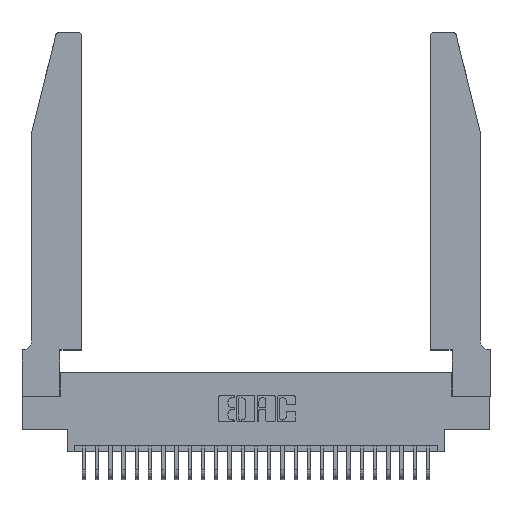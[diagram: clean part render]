
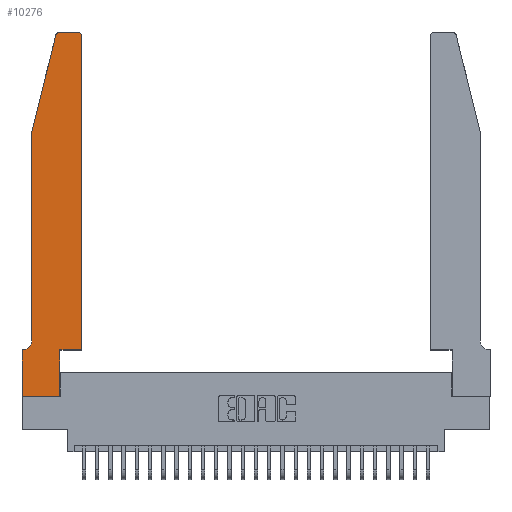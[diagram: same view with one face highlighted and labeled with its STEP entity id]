
A CAD part, top view. The second image highlights one B-rep face of the part: STEP entity #10276.
In plain terms, the highlighted planar face has unit normal (0, 0, 1).
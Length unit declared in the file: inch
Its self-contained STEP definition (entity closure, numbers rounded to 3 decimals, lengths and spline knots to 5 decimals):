
#177 = EDGE_CURVE ( 'NONE', #12363, #7937, #10976, .T. ) ;
#360 = DIRECTION ( 'NONE',  ( 0., -1., 0. ) ) ;
#471 = CARTESIAN_POINT ( 'NONE',  ( 0., 0., 0.37 ) ) ;
#489 = VERTEX_POINT ( 'NONE', #28888 ) ;
#688 = DIRECTION ( 'NONE',  ( -0.239, -0.971, 0. ) ) ;
#980 = EDGE_CURVE ( 'NONE', #6203, #19914, #10920, .T. ) ;
#1013 = CARTESIAN_POINT ( 'NONE',  ( 0., 0., 0.37 ) ) ;
#1745 = CARTESIAN_POINT ( 'NONE',  ( 0.4505, 0.35, 0.37 ) ) ;
#2110 = EDGE_CURVE ( 'NONE', #11754, #8793, #12987, .T. ) ;
#2292 = CARTESIAN_POINT ( 'NONE',  ( 0.0755, 2., 0.37 ) ) ;
#2391 = VERTEX_POINT ( 'NONE', #14574 ) ;
#2503 = VECTOR ( 'NONE', #2788, 39.37008 ) ;
#2513 = ORIENTED_EDGE ( 'NONE', *, *, #2110, .T. ) ;
#2583 = ORIENTED_EDGE ( 'NONE', *, *, #15632, .T. ) ;
#2654 = EDGE_CURVE ( 'NONE', #11881, #7497, #23380, .T. ) ;
#2788 = DIRECTION ( 'NONE',  ( -1., 0., 0. ) ) ;
#2867 = VECTOR ( 'NONE', #21443, 39.37008 ) ;
#3719 = DIRECTION ( 'NONE',  ( 0., 0., 1. ) ) ;
#3841 = CARTESIAN_POINT ( 'NONE',  ( 0.4205, 2.75, 0.37 ) ) ;
#4377 = VECTOR ( 'NONE', #18236, 39.37008 ) ;
#4648 = CARTESIAN_POINT ( 'NONE',  ( 0.284, 2.72, 0.37 ) ) ;
#5442 = DIRECTION ( 'NONE',  ( 1., 0., 0. ) ) ;
#5841 = CARTESIAN_POINT ( 'NONE',  ( 0., 0.35, 0.37 ) ) ;
#6203 = VERTEX_POINT ( 'NONE', #15673 ) ;
#6732 = VECTOR ( 'NONE', #360, 39.37008 ) ;
#6877 = VECTOR ( 'NONE', #18869, 39.37008 ) ;
#7497 = VERTEX_POINT ( 'NONE', #13960 ) ;
#7697 = CARTESIAN_POINT ( 'NONE',  ( 0.0755, 0.42, 0.37 ) ) ;
#7933 = CARTESIAN_POINT ( 'NONE',  ( 0.4205, 2.72, 0.37 ) ) ;
#7937 = VERTEX_POINT ( 'NONE', #13743 ) ;
#8663 = FACE_OUTER_BOUND ( 'NONE', #11438, .T. ) ;
#8793 = VERTEX_POINT ( 'NONE', #24469 ) ;
#9439 = LINE ( 'NONE', #27641, #4377 ) ;
#9674 = DIRECTION ( 'NONE',  ( 0., -1., 0. ) ) ;
#9927 = CARTESIAN_POINT ( 'NONE',  ( 0.4505, 0.35, 0.37 ) ) ;
#9964 = ORIENTED_EDGE ( 'NONE', *, *, #21412, .T. ) ;
#10276 = ADVANCED_FACE ( 'NONE', ( #8663 ), #26796, .T. ) ;
#10920 = LINE ( 'NONE', #14162, #12717 ) ;
#10976 = CIRCLE ( 'NONE', #28673, 0.07 ) ;
#11080 = VERTEX_POINT ( 'NONE', #28340 ) ;
#11148 = ORIENTED_EDGE ( 'NONE', *, *, #28924, .T. ) ;
#11221 = EDGE_CURVE ( 'NONE', #7937, #2391, #26223, .T. ) ;
#11438 = EDGE_LOOP ( 'NONE', ( #2513, #26352, #26016, #28438, #24859, #29668, #17310, #9964, #19159, #11148, #24002, #2583 ) ) ;
#11528 = LINE ( 'NONE', #12059, #2867 ) ;
#11667 = DIRECTION ( 'NONE',  ( 1., 0., 0. ) ) ;
#11708 = DIRECTION ( 'NONE',  ( 0., 0., -1. ) ) ;
#11754 = VERTEX_POINT ( 'NONE', #3841 ) ;
#11881 = VERTEX_POINT ( 'NONE', #9927 ) ;
#11936 = AXIS2_PLACEMENT_3D ( 'NONE', #7933, #19351, #29120 ) ;
#12022 = CARTESIAN_POINT ( 'NONE',  ( 0.2605, 2.75, 0.37 ) ) ;
#12059 = CARTESIAN_POINT ( 'NONE',  ( 0.4505, 0.35, 0.37 ) ) ;
#12363 = VERTEX_POINT ( 'NONE', #7697 ) ;
#12428 = CIRCLE ( 'NONE', #14003, 0.03 ) ;
#12717 = VECTOR ( 'NONE', #688, 39.37008 ) ;
#12831 = LINE ( 'NONE', #471, #6732 ) ;
#12987 = LINE ( 'NONE', #12022, #6877 ) ;
#13413 = EDGE_CURVE ( 'NONE', #8793, #6203, #12428, .T. ) ;
#13743 = CARTESIAN_POINT ( 'NONE',  ( 0.0055, 0.35, 0.37 ) ) ;
#13960 = CARTESIAN_POINT ( 'NONE',  ( 0.4505, 2.72, 0.37 ) ) ;
#14003 = AXIS2_PLACEMENT_3D ( 'NONE', #4648, #18229, #11667 ) ;
#14131 = DIRECTION ( 'NONE',  ( -1., 0., 0. ) ) ;
#14162 = CARTESIAN_POINT ( 'NONE',  ( 0.0755, 2., 0.37 ) ) ;
#14574 = CARTESIAN_POINT ( 'NONE',  ( 0., 0.35, 0.37 ) ) ;
#15402 = EDGE_CURVE ( 'NONE', #25795, #11080, #9439, .T. ) ;
#15632 = EDGE_CURVE ( 'NONE', #7497, #11754, #22418, .T. ) ;
#15673 = CARTESIAN_POINT ( 'NONE',  ( 0.25487, 2.72718, 0.37 ) ) ;
#16057 = CARTESIAN_POINT ( 'NONE',  ( 0.0055, 0.42, 0.37 ) ) ;
#16562 = CARTESIAN_POINT ( 'NONE',  ( 0.0755, 0.35, 0.37 ) ) ;
#16608 = LINE ( 'NONE', #1013, #21671 ) ;
#17310 = ORIENTED_EDGE ( 'NONE', *, *, #24957, .T. ) ;
#17913 = CARTESIAN_POINT ( 'NONE',  ( 0.2865, 0., 0.37 ) ) ;
#18229 = DIRECTION ( 'NONE',  ( 0., 0., 1. ) ) ;
#18236 = DIRECTION ( 'NONE',  ( 0., 1., 0. ) ) ;
#18338 = LINE ( 'NONE', #25824, #28359 ) ;
#18869 = DIRECTION ( 'NONE',  ( -1., 0., 0. ) ) ;
#19159 = ORIENTED_EDGE ( 'NONE', *, *, #15402, .T. ) ;
#19351 = DIRECTION ( 'NONE',  ( 0., 0., 1. ) ) ;
#19914 = VERTEX_POINT ( 'NONE', #2292 ) ;
#21412 = EDGE_CURVE ( 'NONE', #489, #25795, #16608, .T. ) ;
#21443 = DIRECTION ( 'NONE',  ( 1., 0., 0. ) ) ;
#21671 = VECTOR ( 'NONE', #5442, 39.37008 ) ;
#22418 = CIRCLE ( 'NONE', #11936, 0.03 ) ;
#22507 = EDGE_CURVE ( 'NONE', #19914, #12363, #18338, .T. ) ;
#23380 = LINE ( 'NONE', #1745, #27680 ) ;
#24002 = ORIENTED_EDGE ( 'NONE', *, *, #2654, .T. ) ;
#24469 = CARTESIAN_POINT ( 'NONE',  ( 0.284, 2.75, 0.37 ) ) ;
#24859 = ORIENTED_EDGE ( 'NONE', *, *, #177, .T. ) ;
#24957 = EDGE_CURVE ( 'NONE', #2391, #489, #12831, .T. ) ;
#25778 = AXIS2_PLACEMENT_3D ( 'NONE', #5841, #3719, #28824 ) ;
#25795 = VERTEX_POINT ( 'NONE', #17913 ) ;
#25824 = CARTESIAN_POINT ( 'NONE',  ( 0.0755, 2., 0.37 ) ) ;
#26016 = ORIENTED_EDGE ( 'NONE', *, *, #980, .T. ) ;
#26223 = LINE ( 'NONE', #16562, #2503 ) ;
#26352 = ORIENTED_EDGE ( 'NONE', *, *, #13413, .T. ) ;
#26796 = PLANE ( 'NONE',  #25778 ) ;
#27641 = CARTESIAN_POINT ( 'NONE',  ( 0.2865, 0.35, 0.37 ) ) ;
#27680 = VECTOR ( 'NONE', #29145, 39.37008 ) ;
#28340 = CARTESIAN_POINT ( 'NONE',  ( 0.2865, 0.35, 0.37 ) ) ;
#28359 = VECTOR ( 'NONE', #9674, 39.37008 ) ;
#28438 = ORIENTED_EDGE ( 'NONE', *, *, #22507, .T. ) ;
#28673 = AXIS2_PLACEMENT_3D ( 'NONE', #16057, #11708, #14131 ) ;
#28824 = DIRECTION ( 'NONE',  ( 1., 0., 0. ) ) ;
#28888 = CARTESIAN_POINT ( 'NONE',  ( 0., 0., 0.37 ) ) ;
#28924 = EDGE_CURVE ( 'NONE', #11080, #11881, #11528, .T. ) ;
#29120 = DIRECTION ( 'NONE',  ( 1., 0., 0. ) ) ;
#29145 = DIRECTION ( 'NONE',  ( 0., 1., 0. ) ) ;
#29668 = ORIENTED_EDGE ( 'NONE', *, *, #11221, .T. ) ;
